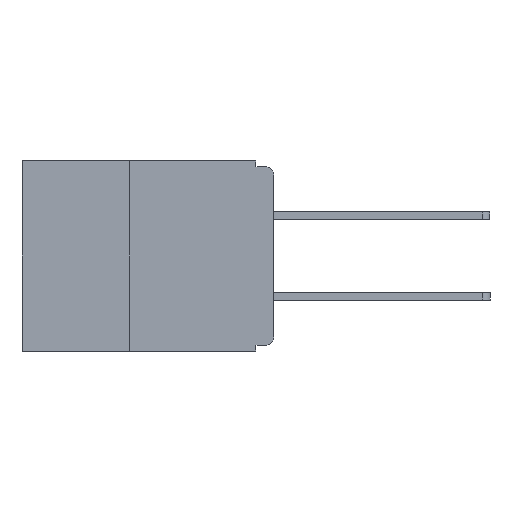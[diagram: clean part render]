
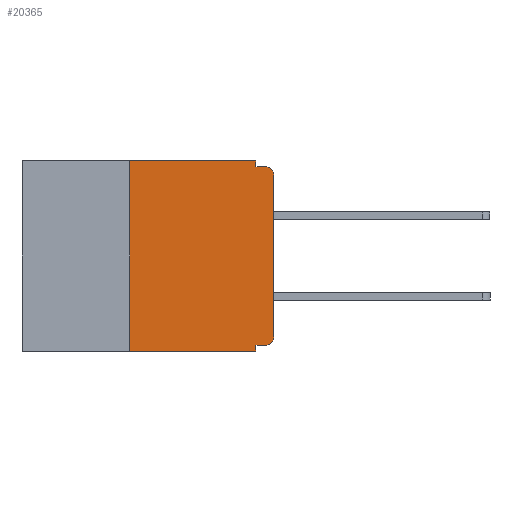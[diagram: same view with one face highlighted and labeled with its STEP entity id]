
A CAD part, left-side view. The second image highlights one B-rep face of the part: STEP entity #20365.
In plain terms, the highlighted planar face has unit normal (-1, 0, 0).
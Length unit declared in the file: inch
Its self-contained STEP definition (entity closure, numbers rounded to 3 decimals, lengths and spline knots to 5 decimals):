
#32 = ORIENTED_EDGE ( 'NONE', *, *, #1212, .T. ) ;
#54 = DIRECTION ( 'NONE',  ( 0., -1., 0. ) ) ;
#326 = ORIENTED_EDGE ( 'NONE', *, *, #5932, .F. ) ;
#823 = LINE ( 'NONE', #21319, #9836 ) ;
#910 = DIRECTION ( 'NONE',  ( 0., -1., 0. ) ) ;
#1212 = EDGE_CURVE ( 'NONE', #7464, #13079, #12359, .T. ) ;
#1551 = VECTOR ( 'NONE', #910, 39.37008 ) ;
#2124 = VECTOR ( 'NONE', #14155, 39.37008 ) ;
#2294 = VERTEX_POINT ( 'NONE', #17163 ) ;
#2661 = CARTESIAN_POINT ( 'NONE',  ( 0., 0.25, -0.33 ) ) ;
#2751 = CARTESIAN_POINT ( 'NONE',  ( 0., 0.437, -0.33 ) ) ;
#2768 = EDGE_LOOP ( 'NONE', ( #10757, #17119, #21667, #13000, #22742, #326, #16861, #21426, #12735, #32 ) ) ;
#3276 = VECTOR ( 'NONE', #12338, 39.37008 ) ;
#3288 = CARTESIAN_POINT ( 'NONE',  ( 0., 0.437, 0. ) ) ;
#3499 = PLANE ( 'NONE',  #6716 ) ;
#3559 = VERTEX_POINT ( 'NONE', #13888 ) ;
#3806 = LINE ( 'NONE', #13967, #17407 ) ;
#3840 = CARTESIAN_POINT ( 'NONE',  ( 0., 0.25, 0. ) ) ;
#5236 = CARTESIAN_POINT ( 'NONE',  ( 0., 0.437, 0. ) ) ;
#5321 = DIRECTION ( 'NONE',  ( 0., 0., -1. ) ) ;
#5932 = EDGE_CURVE ( 'NONE', #6284, #22095, #15807, .T. ) ;
#6123 = DIRECTION ( 'NONE',  ( 0., 1., 0. ) ) ;
#6284 = VERTEX_POINT ( 'NONE', #2661 ) ;
#6716 = AXIS2_PLACEMENT_3D ( 'NONE', #5236, #15963, #5321 ) ;
#6841 = CARTESIAN_POINT ( 'NONE',  ( 0., 0.015, -0.025 ) ) ;
#7464 = VERTEX_POINT ( 'NONE', #12133 ) ;
#7487 = LINE ( 'NONE', #2751, #1551 ) ;
#7734 = DIRECTION ( 'NONE',  ( 0., 0., -1. ) ) ;
#8440 = VERTEX_POINT ( 'NONE', #11163 ) ;
#8681 = DIRECTION ( 'NONE',  ( 0., 0., -1. ) ) ;
#9075 = VECTOR ( 'NONE', #6123, 39.37008 ) ;
#9293 = CARTESIAN_POINT ( 'NONE',  ( 0., 0.031, 0. ) ) ;
#9746 = AXIS2_PLACEMENT_3D ( 'NONE', #6841, #19192, #8681 ) ;
#9836 = VECTOR ( 'NONE', #54, 39.37008 ) ;
#10144 = LINE ( 'NONE', #11433, #9075 ) ;
#10150 = EDGE_CURVE ( 'NONE', #7464, #17697, #10144, .T. ) ;
#10493 = VECTOR ( 'NONE', #12604, 39.37008 ) ;
#10633 = EDGE_CURVE ( 'NONE', #6284, #17496, #7487, .T. ) ;
#10757 = ORIENTED_EDGE ( 'NONE', *, *, #16739, .T. ) ;
#11163 = CARTESIAN_POINT ( 'NONE',  ( 0., 0.031, 0. ) ) ;
#11433 = CARTESIAN_POINT ( 'NONE',  ( 0., 0., -0.32 ) ) ;
#11481 = VECTOR ( 'NONE', #13950, 39.37008 ) ;
#11684 = EDGE_CURVE ( 'NONE', #2294, #3559, #15074, .T. ) ;
#11984 = CARTESIAN_POINT ( 'NONE',  ( 0., 0.015, -0.305 ) ) ;
#12102 = DIRECTION ( 'NONE',  ( -1., 0., 0. ) ) ;
#12133 = CARTESIAN_POINT ( 'NONE',  ( 0., 0.015, -0.32 ) ) ;
#12265 = DIRECTION ( 'NONE',  ( 0., 0., 1. ) ) ;
#12338 = DIRECTION ( 'NONE',  ( 0., 0., -1. ) ) ;
#12359 = CIRCLE ( 'NONE', #17990, 0.015 ) ;
#12604 = DIRECTION ( 'NONE',  ( 0., 0., -1. ) ) ;
#12735 = ORIENTED_EDGE ( 'NONE', *, *, #10150, .F. ) ;
#13000 = ORIENTED_EDGE ( 'NONE', *, *, #14988, .F. ) ;
#13015 = CARTESIAN_POINT ( 'NONE',  ( 0., 0.031, -0.32 ) ) ;
#13079 = VERTEX_POINT ( 'NONE', #17621 ) ;
#13577 = EDGE_CURVE ( 'NONE', #17697, #17496, #17462, .T. ) ;
#13888 = CARTESIAN_POINT ( 'NONE',  ( 0., 0.015, -0.01 ) ) ;
#13950 = DIRECTION ( 'NONE',  ( 0., -1., 0. ) ) ;
#13967 = CARTESIAN_POINT ( 'NONE',  ( 0., 0., 0. ) ) ;
#14155 = DIRECTION ( 'NONE',  ( 0., 0., 1. ) ) ;
#14787 = FACE_OUTER_BOUND ( 'NONE', #2768, .T. ) ;
#14988 = EDGE_CURVE ( 'NONE', #8440, #17583, #15221, .T. ) ;
#15074 = CIRCLE ( 'NONE', #9746, 0.015 ) ;
#15221 = LINE ( 'NONE', #9293, #10493 ) ;
#15807 = LINE ( 'NONE', #22754, #2124 ) ;
#15963 = DIRECTION ( 'NONE',  ( 1., 0., 0. ) ) ;
#16207 = LINE ( 'NONE', #3288, #11481 ) ;
#16739 = EDGE_CURVE ( 'NONE', #13079, #2294, #3806, .T. ) ;
#16861 = ORIENTED_EDGE ( 'NONE', *, *, #10633, .T. ) ;
#17119 = ORIENTED_EDGE ( 'NONE', *, *, #11684, .T. ) ;
#17163 = CARTESIAN_POINT ( 'NONE',  ( 0., 0., -0.025 ) ) ;
#17407 = VECTOR ( 'NONE', #12265, 39.37008 ) ;
#17462 = LINE ( 'NONE', #19312, #3276 ) ;
#17496 = VERTEX_POINT ( 'NONE', #22924 ) ;
#17583 = VERTEX_POINT ( 'NONE', #21364 ) ;
#17621 = CARTESIAN_POINT ( 'NONE',  ( 0., 0., -0.305 ) ) ;
#17697 = VERTEX_POINT ( 'NONE', #13015 ) ;
#17990 = AXIS2_PLACEMENT_3D ( 'NONE', #11984, #12102, #7734 ) ;
#19192 = DIRECTION ( 'NONE',  ( -1., 0., 0. ) ) ;
#19312 = CARTESIAN_POINT ( 'NONE',  ( 0., 0.031, -0.33 ) ) ;
#19355 = EDGE_CURVE ( 'NONE', #17583, #3559, #823, .T. ) ;
#19705 = EDGE_CURVE ( 'NONE', #22095, #8440, #16207, .T. ) ;
#20365 = ADVANCED_FACE ( 'NONE', ( #14787 ), #3499, .F. ) ;
#21319 = CARTESIAN_POINT ( 'NONE',  ( 0., 0., -0.01 ) ) ;
#21364 = CARTESIAN_POINT ( 'NONE',  ( 0., 0.031, -0.01 ) ) ;
#21426 = ORIENTED_EDGE ( 'NONE', *, *, #13577, .F. ) ;
#21667 = ORIENTED_EDGE ( 'NONE', *, *, #19355, .F. ) ;
#22095 = VERTEX_POINT ( 'NONE', #3840 ) ;
#22742 = ORIENTED_EDGE ( 'NONE', *, *, #19705, .F. ) ;
#22754 = CARTESIAN_POINT ( 'NONE',  ( 0., 0.25, -0.33 ) ) ;
#22924 = CARTESIAN_POINT ( 'NONE',  ( 0., 0.031, -0.33 ) ) ;
